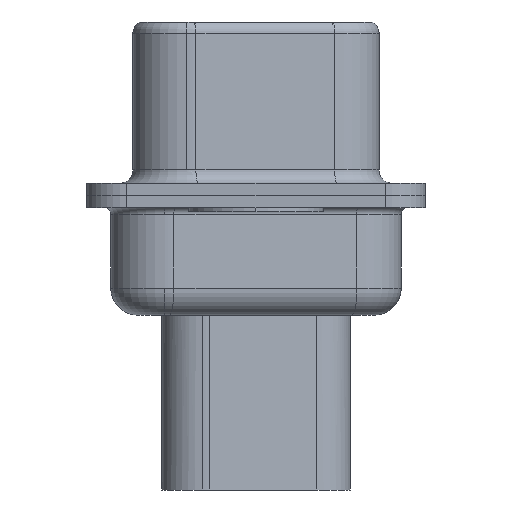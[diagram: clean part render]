
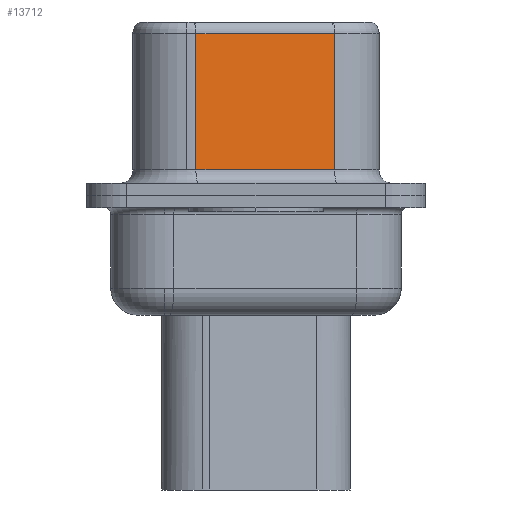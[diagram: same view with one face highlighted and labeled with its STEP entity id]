
A CAD part, left-side view. The second image highlights one B-rep face of the part: STEP entity #13712.
In plain terms, the highlighted planar face has unit normal (-0.985, -0.174, 0).
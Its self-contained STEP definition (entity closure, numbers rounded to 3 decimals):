
#437 = DIRECTION ( 'NONE',  ( 0., 0., -1. ) ) ;
#1258 = VERTEX_POINT ( 'NONE', #20043 ) ;
#1802 = EDGE_CURVE ( 'NONE', #19860, #6449, #3868, .T. ) ;
#2083 = CARTESIAN_POINT ( 'NONE',  ( 4.58, -2.927, 6.52 ) ) ;
#3486 = LINE ( 'NONE', #5443, #10822 ) ;
#3662 = DIRECTION ( 'NONE',  ( 0., 0., -1. ) ) ;
#3868 = LINE ( 'NONE', #8688, #7861 ) ;
#4181 = CARTESIAN_POINT ( 'NONE',  ( 4.58, -2.927, 6.52 ) ) ;
#5443 = CARTESIAN_POINT ( 'NONE',  ( 4.58, -2.927, 6.02 ) ) ;
#6449 = VERTEX_POINT ( 'NONE', #10788 ) ;
#6867 = ORIENTED_EDGE ( 'NONE', *, *, #10411, .F. ) ;
#7064 = FACE_OUTER_BOUND ( 'NONE', #9319, .T. ) ;
#7861 = VECTOR ( 'NONE', #10333, 1000. ) ;
#8263 = ORIENTED_EDGE ( 'NONE', *, *, #9995, .T. ) ;
#8492 = PLANE ( 'NONE',  #14450 ) ;
#8688 = CARTESIAN_POINT ( 'NONE',  ( 4.58, -2.927, 0.95 ) ) ;
#9319 = EDGE_LOOP ( 'NONE', ( #6867, #10477, #8263, #11002 ) ) ;
#9995 = EDGE_CURVE ( 'NONE', #14917, #19860, #14554, .T. ) ;
#10333 = DIRECTION ( 'NONE',  ( 0.174, -0.985, 0. ) ) ;
#10411 = EDGE_CURVE ( 'NONE', #1258, #6449, #16281, .T. ) ;
#10477 = ORIENTED_EDGE ( 'NONE', *, *, #11285, .T. ) ;
#10788 = CARTESIAN_POINT ( 'NONE',  ( 4.58, -2.927, 0.95 ) ) ;
#10822 = VECTOR ( 'NONE', #18170, 1000. ) ;
#11002 = ORIENTED_EDGE ( 'NONE', *, *, #1802, .T. ) ;
#11285 = EDGE_CURVE ( 'NONE', #1258, #14917, #3486, .T. ) ;
#11367 = CARTESIAN_POINT ( 'NONE',  ( 3.67, 2.233, 6.52 ) ) ;
#13247 = CARTESIAN_POINT ( 'NONE',  ( 3.67, 2.233, 6.02 ) ) ;
#13712 = ADVANCED_FACE ( 'NONE', ( #7064 ), #8492, .F. ) ;
#14450 = AXIS2_PLACEMENT_3D ( 'NONE', #4181, #18161, #18355 ) ;
#14554 = LINE ( 'NONE', #11367, #16033 ) ;
#14917 = VERTEX_POINT ( 'NONE', #13247 ) ;
#16033 = VECTOR ( 'NONE', #3662, 1000. ) ;
#16281 = LINE ( 'NONE', #2083, #16384 ) ;
#16384 = VECTOR ( 'NONE', #437, 1000. ) ;
#16394 = CARTESIAN_POINT ( 'NONE',  ( 3.67, 2.233, 0.95 ) ) ;
#18161 = DIRECTION ( 'NONE',  ( 0.985, 0.174, 0. ) ) ;
#18170 = DIRECTION ( 'NONE',  ( -0.174, 0.985, 0. ) ) ;
#18355 = DIRECTION ( 'NONE',  ( -0.174, 0.985, 0. ) ) ;
#19860 = VERTEX_POINT ( 'NONE', #16394 ) ;
#20043 = CARTESIAN_POINT ( 'NONE',  ( 4.58, -2.927, 6.02 ) ) ;
